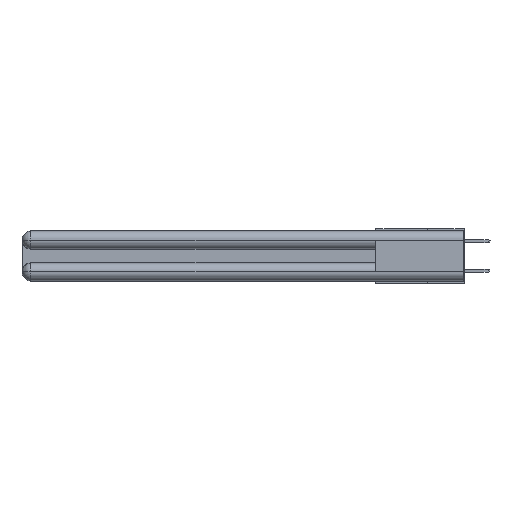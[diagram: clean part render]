
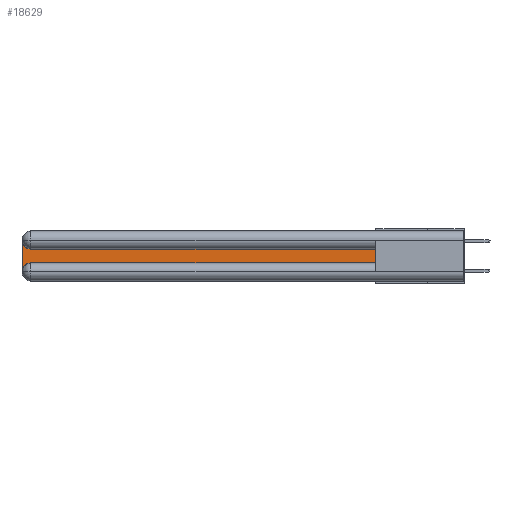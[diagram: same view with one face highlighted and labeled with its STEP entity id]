
A CAD part, left-side view. The second image highlights one B-rep face of the part: STEP entity #18629.
In plain terms, the highlighted planar face has unit normal (-1, 0, 0).
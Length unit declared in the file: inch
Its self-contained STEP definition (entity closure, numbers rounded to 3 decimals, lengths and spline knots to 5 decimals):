
#28 = DIRECTION ( 'NONE',  ( 0., 0., -1. ) ) ;
#119 = CARTESIAN_POINT ( 'NONE',  ( 0.075, 0.6, -0.1225 ) ) ;
#1526 = EDGE_CURVE ( 'NONE', #13390, #24428, #21169, .T. ) ;
#1872 = ORIENTED_EDGE ( 'NONE', *, *, #25328, .T. ) ;
#2363 = DIRECTION ( 'NONE',  ( 0., -1., 0. ) ) ;
#2389 = ORIENTED_EDGE ( 'NONE', *, *, #25372, .T. ) ;
#2490 = CARTESIAN_POINT ( 'NONE',  ( 0.075, 2.94, -0.0625 ) ) ;
#3988 = DIRECTION ( 'NONE',  ( 1., 0., 0. ) ) ;
#4091 = CARTESIAN_POINT ( 'NONE',  ( 0.075, 3., -0.2175 ) ) ;
#4163 = ORIENTED_EDGE ( 'NONE', *, *, #26050, .T. ) ;
#4493 = DIRECTION ( 'NONE',  ( 1., 0., 0. ) ) ;
#4754 = CARTESIAN_POINT ( 'NONE',  ( 0.075, 2.94, -0.2775 ) ) ;
#5328 = CARTESIAN_POINT ( 'NONE',  ( 0.075, 0.6, -0.1225 ) ) ;
#5438 = CARTESIAN_POINT ( 'NONE',  ( 0.075, 2.94, -0.2175 ) ) ;
#6242 = VECTOR ( 'NONE', #15444, 39.37008 ) ;
#6465 = DIRECTION ( 'NONE',  ( 0., 0., -1. ) ) ;
#7030 = CARTESIAN_POINT ( 'NONE',  ( 0.075, 0.6, -0.2175 ) ) ;
#7866 = EDGE_CURVE ( 'NONE', #24428, #32011, #21525, .T. ) ;
#8074 = CARTESIAN_POINT ( 'NONE',  ( 0.075, 3., -0.2775 ) ) ;
#8918 = DIRECTION ( 'NONE',  ( 0., 0., 1. ) ) ;
#9037 = ORIENTED_EDGE ( 'NONE', *, *, #1526, .T. ) ;
#9836 = DIRECTION ( 'NONE',  ( 1., 0., 0. ) ) ;
#13390 = VERTEX_POINT ( 'NONE', #5328 ) ;
#13735 = AXIS2_PLACEMENT_3D ( 'NONE', #30139, #9836, #30246 ) ;
#13993 = CARTESIAN_POINT ( 'NONE',  ( 0.075, 0.6, -0.2175 ) ) ;
#14438 = LINE ( 'NONE', #13993, #20100 ) ;
#15035 = EDGE_CURVE ( 'NONE', #29093, #13390, #14438, .T. ) ;
#15164 = PLANE ( 'NONE',  #13735 ) ;
#15444 = DIRECTION ( 'NONE',  ( 0., 1., 0. ) ) ;
#17215 = CIRCLE ( 'NONE', #27442, 0.06 ) ;
#17809 = CARTESIAN_POINT ( 'NONE',  ( 0.075, 0.6, -0.2175 ) ) ;
#18368 = VECTOR ( 'NONE', #2363, 39.37008 ) ;
#18629 = ADVANCED_FACE ( 'NONE', ( #25059 ), #15164, .F. ) ;
#18840 = VERTEX_POINT ( 'NONE', #5438 ) ;
#20100 = VECTOR ( 'NONE', #8918, 39.37008 ) ;
#20670 = AXIS2_PLACEMENT_3D ( 'NONE', #2490, #4493, #28 ) ;
#21169 = LINE ( 'NONE', #119, #6242 ) ;
#21525 = CIRCLE ( 'NONE', #20670, 0.06 ) ;
#21644 = VECTOR ( 'NONE', #32932, 39.37008 ) ;
#22200 = CARTESIAN_POINT ( 'NONE',  ( 0.075, 3., -0.0625 ) ) ;
#23920 = VERTEX_POINT ( 'NONE', #8074 ) ;
#24428 = VERTEX_POINT ( 'NONE', #30001 ) ;
#25059 = FACE_OUTER_BOUND ( 'NONE', #25390, .T. ) ;
#25328 = EDGE_CURVE ( 'NONE', #23920, #18840, #17215, .T. ) ;
#25372 = EDGE_CURVE ( 'NONE', #32011, #23920, #31702, .T. ) ;
#25390 = EDGE_LOOP ( 'NONE', ( #9037, #29893, #2389, #1872, #4163, #31618 ) ) ;
#26050 = EDGE_CURVE ( 'NONE', #18840, #29093, #30436, .T. ) ;
#27442 = AXIS2_PLACEMENT_3D ( 'NONE', #4754, #3988, #6465 ) ;
#29093 = VERTEX_POINT ( 'NONE', #7030 ) ;
#29893 = ORIENTED_EDGE ( 'NONE', *, *, #7866, .T. ) ;
#30001 = CARTESIAN_POINT ( 'NONE',  ( 0.075, 2.94, -0.1225 ) ) ;
#30139 = CARTESIAN_POINT ( 'NONE',  ( 0.075, 3., -0.1225 ) ) ;
#30246 = DIRECTION ( 'NONE',  ( 0., 0., -1. ) ) ;
#30436 = LINE ( 'NONE', #17809, #18368 ) ;
#31618 = ORIENTED_EDGE ( 'NONE', *, *, #15035, .T. ) ;
#31702 = LINE ( 'NONE', #4091, #21644 ) ;
#32011 = VERTEX_POINT ( 'NONE', #22200 ) ;
#32932 = DIRECTION ( 'NONE',  ( 0., 0., -1. ) ) ;
